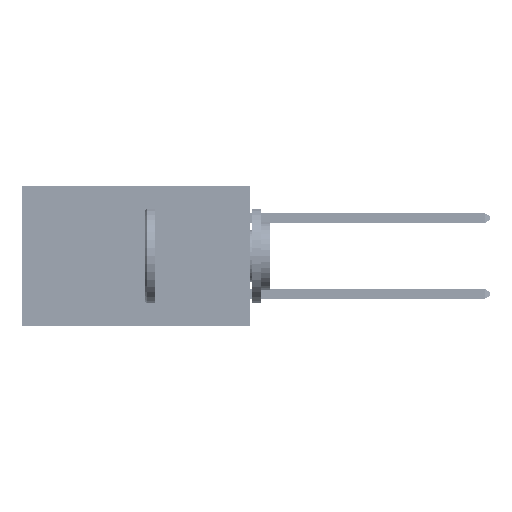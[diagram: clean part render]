
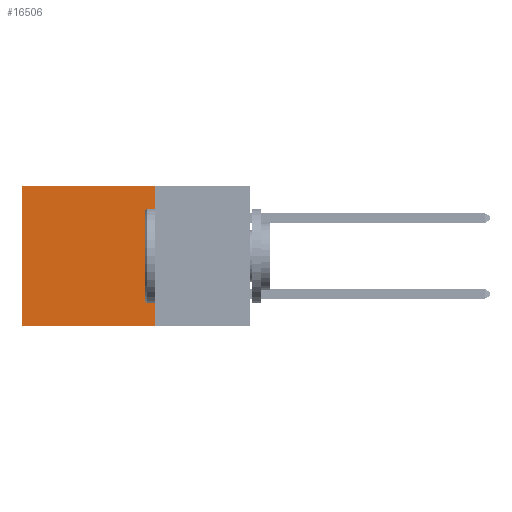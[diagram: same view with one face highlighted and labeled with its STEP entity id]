
A CAD part, left-side view. The second image highlights one B-rep face of the part: STEP entity #16506.
In plain terms, the highlighted planar face has unit normal (-1, 0, 0).
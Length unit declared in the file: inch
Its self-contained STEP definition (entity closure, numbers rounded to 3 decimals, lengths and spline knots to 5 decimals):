
#148 = VECTOR ( 'NONE', #3730, 39.37008 ) ;
#1108 = ORIENTED_EDGE ( 'NONE', *, *, #48018, .F. ) ;
#2675 = CARTESIAN_POINT ( 'NONE',  ( 0.2875, 0.25, 0. ) ) ;
#3730 = DIRECTION ( 'NONE',  ( 0., 1., 0. ) ) ;
#6464 = LINE ( 'NONE', #36656, #35247 ) ;
#6511 = PLANE ( 'NONE',  #39299 ) ;
#9357 = VECTOR ( 'NONE', #31381, 39.37008 ) ;
#11413 = EDGE_CURVE ( 'NONE', #46714, #12152, #21501, .T. ) ;
#12152 = VERTEX_POINT ( 'NONE', #45680 ) ;
#12200 = VERTEX_POINT ( 'NONE', #27272 ) ;
#13964 = EDGE_LOOP ( 'NONE', ( #26545, #26797, #1108, #31121 ) ) ;
#14142 = DIRECTION ( 'NONE',  ( 0., 0., -1. ) ) ;
#16506 = ADVANCED_FACE ( 'NONE', ( #29102 ), #6511, .F. ) ;
#20658 = LINE ( 'NONE', #37318, #39356 ) ;
#21501 = LINE ( 'NONE', #37991, #148 ) ;
#23902 = CARTESIAN_POINT ( 'NONE',  ( 0.2875, 0.6, 0. ) ) ;
#26545 = ORIENTED_EDGE ( 'NONE', *, *, #43322, .T. ) ;
#26797 = ORIENTED_EDGE ( 'NONE', *, *, #47897, .F. ) ;
#27272 = CARTESIAN_POINT ( 'NONE',  ( 0.2875, 0.25, -0.37 ) ) ;
#29102 = FACE_OUTER_BOUND ( 'NONE', #13964, .T. ) ;
#31121 = ORIENTED_EDGE ( 'NONE', *, *, #11413, .T. ) ;
#31381 = DIRECTION ( 'NONE',  ( 0., 0., -1. ) ) ;
#32908 = DIRECTION ( 'NONE',  ( 0., 1., 0. ) ) ;
#33988 = CARTESIAN_POINT ( 'NONE',  ( 0.2875, 0.25, 0. ) ) ;
#35247 = VECTOR ( 'NONE', #32908, 39.37008 ) ;
#36541 = DIRECTION ( 'NONE',  ( 1., 0., 0. ) ) ;
#36656 = CARTESIAN_POINT ( 'NONE',  ( 0.2875, 0.25, -0.37 ) ) ;
#37318 = CARTESIAN_POINT ( 'NONE',  ( 0.2875, 0.25, 0. ) ) ;
#37991 = CARTESIAN_POINT ( 'NONE',  ( 0.2875, 0.25, 0. ) ) ;
#39299 = AXIS2_PLACEMENT_3D ( 'NONE', #2675, #36541, #14142 ) ;
#39300 = LINE ( 'NONE', #23902, #9357 ) ;
#39356 = VECTOR ( 'NONE', #40927, 39.37008 ) ;
#40927 = DIRECTION ( 'NONE',  ( 0., 0., -1. ) ) ;
#42296 = VERTEX_POINT ( 'NONE', #47438 ) ;
#43322 = EDGE_CURVE ( 'NONE', #12152, #42296, #39300, .T. ) ;
#45680 = CARTESIAN_POINT ( 'NONE',  ( 0.2875, 0.6, 0. ) ) ;
#46714 = VERTEX_POINT ( 'NONE', #33988 ) ;
#47438 = CARTESIAN_POINT ( 'NONE',  ( 0.2875, 0.6, -0.37 ) ) ;
#47897 = EDGE_CURVE ( 'NONE', #12200, #42296, #6464, .T. ) ;
#48018 = EDGE_CURVE ( 'NONE', #46714, #12200, #20658, .T. ) ;
